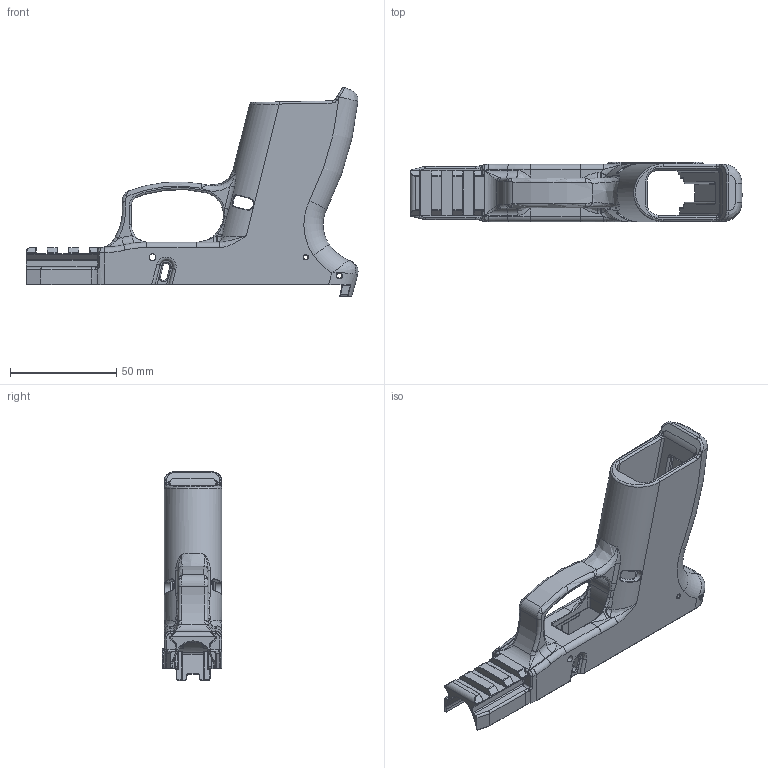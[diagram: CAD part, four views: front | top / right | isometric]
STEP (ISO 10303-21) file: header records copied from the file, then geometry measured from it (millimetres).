
FILE_DESCRIPTION(/* description */ (''),/* implementation_level */ '2;1');
FILE_NAME(/* name */ 'FOSS-CANNON-v1.1.step',/* time_stamp */ '2022-02-09T15:29:37-08:00',/* author */ (''),/* organization */ (''),/* preprocessor_version */ 'ST-DEVELOPER v18.1',/* originating_system */ 'Autodesk Translation Framework v10.13.0.1454',/* authorisation */ '');
FILE_SCHEMA (('AUTOMOTIVE_DESIGN { 1 0 10303 214 3 1 1 }'));
Products named in the file (1): (Unsaved)
Bounding box: 156.07 x 28 x 98.27 mm (x, y, z)
Volume: 67868.5 mm3; surface area: 37009.5 mm2
Topology: 1 solids, 1 shells, 1265 faces, 3424 edges, 2075 vertices
Faces by surface type: cylinder 490, bspline 310, torus 234, plane 194, cone 22, sphere 15
Full cylindrical faces by diameter (mm): 2 x2, 2.5 x2, 3.2 x2
Entity records: 54364 total; most frequent: CARTESIAN_POINT 24380, ORIENTED_EDGE 6692, DIRECTION 5931, EDGE_CURVE 3346, AXIS2_PLACEMENT_3D 2440, VERTEX_POINT 2073, EDGE_LOOP 1281, FACE_OUTER_BOUND 1265
